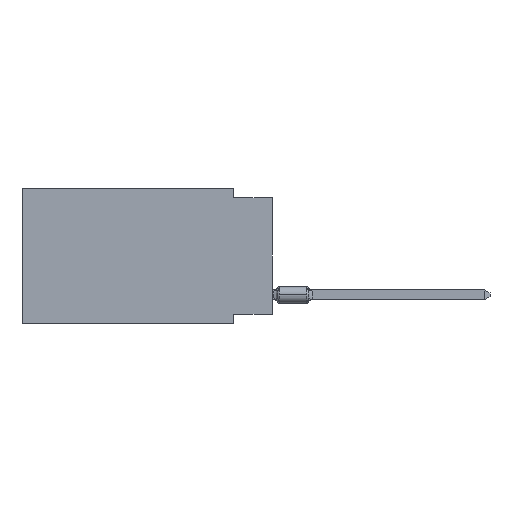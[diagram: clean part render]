
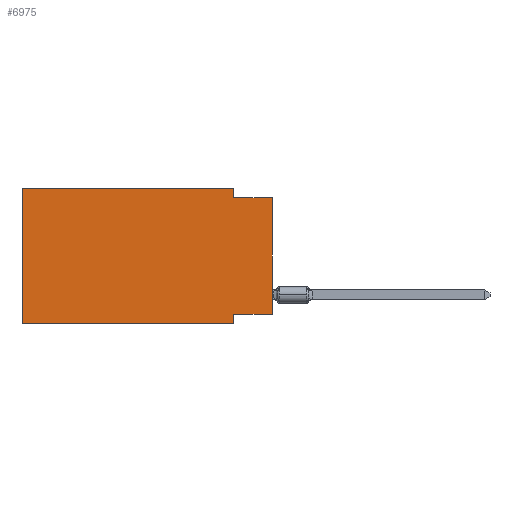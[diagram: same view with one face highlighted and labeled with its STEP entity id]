
A CAD part, left-side view. The second image highlights one B-rep face of the part: STEP entity #6975.
In plain terms, the highlighted planar face has unit normal (-1, 0, 0).
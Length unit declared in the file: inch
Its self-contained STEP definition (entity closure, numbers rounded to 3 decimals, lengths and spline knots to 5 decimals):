
#52 = DIRECTION ( 'NONE',  ( 0., 0., -1. ) ) ;
#82 = CARTESIAN_POINT ( 'NONE',  ( 0., 0.645, -0.35 ) ) ;
#137 = CARTESIAN_POINT ( 'NONE',  ( 0., 0., -0.025 ) ) ;
#347 = VECTOR ( 'NONE', #8689, 39.37008 ) ;
#654 = ORIENTED_EDGE ( 'NONE', *, *, #1019, .T. ) ;
#714 = EDGE_CURVE ( 'NONE', #12337, #725, #11380, .T. ) ;
#725 = VERTEX_POINT ( 'NONE', #10423 ) ;
#746 = VECTOR ( 'NONE', #10069, 39.37008 ) ;
#795 = VECTOR ( 'NONE', #7187, 39.37008 ) ;
#1019 = EDGE_CURVE ( 'NONE', #2766, #12699, #1999, .T. ) ;
#1235 = ORIENTED_EDGE ( 'NONE', *, *, #10185, .F. ) ;
#1402 = EDGE_LOOP ( 'NONE', ( #654, #4165, #5608, #5534, #11131, #13465, #12057, #1235 ) ) ;
#1779 = VERTEX_POINT ( 'NONE', #12945 ) ;
#1970 = EDGE_CURVE ( 'NONE', #10021, #12699, #12278, .T. ) ;
#1999 = LINE ( 'NONE', #2071, #795 ) ;
#2071 = CARTESIAN_POINT ( 'NONE',  ( 0., 0., 0. ) ) ;
#2283 = CARTESIAN_POINT ( 'NONE',  ( 0., 0.645, 0. ) ) ;
#2307 = VECTOR ( 'NONE', #9966, 39.37008 ) ;
#2342 = LINE ( 'NONE', #7653, #347 ) ;
#2606 = CARTESIAN_POINT ( 'NONE',  ( 0., 0.1, 0. ) ) ;
#2766 = VERTEX_POINT ( 'NONE', #10666 ) ;
#3580 = DIRECTION ( 'NONE',  ( 0., -1., 0. ) ) ;
#4165 = ORIENTED_EDGE ( 'NONE', *, *, #1970, .F. ) ;
#4699 = DIRECTION ( 'NONE',  ( 0., 1., 0. ) ) ;
#5534 = ORIENTED_EDGE ( 'NONE', *, *, #10405, .F. ) ;
#5608 = ORIENTED_EDGE ( 'NONE', *, *, #10258, .F. ) ;
#5720 = EDGE_CURVE ( 'NONE', #12337, #11978, #7946, .T. ) ;
#5856 = CARTESIAN_POINT ( 'NONE',  ( 0., 0.1, 0. ) ) ;
#5901 = CARTESIAN_POINT ( 'NONE',  ( 0., 0.645, -0.35 ) ) ;
#5912 = VERTEX_POINT ( 'NONE', #2606 ) ;
#5913 = LINE ( 'NONE', #7006, #7324 ) ;
#5996 = VECTOR ( 'NONE', #10351, 39.37008 ) ;
#6123 = CARTESIAN_POINT ( 'NONE',  ( 0., 0., -0.025 ) ) ;
#6245 = DIRECTION ( 'NONE',  ( 1., 0., 0. ) ) ;
#6637 = CARTESIAN_POINT ( 'NONE',  ( 0., 0.645, 0. ) ) ;
#6774 = LINE ( 'NONE', #6637, #11492 ) ;
#6975 = ADVANCED_FACE ( 'NONE', ( #7466 ), #11645, .F. ) ;
#7006 = CARTESIAN_POINT ( 'NONE',  ( 0., 0., -0.325 ) ) ;
#7187 = DIRECTION ( 'NONE',  ( 0., 0., 1. ) ) ;
#7324 = VECTOR ( 'NONE', #4699, 39.37008 ) ;
#7466 = FACE_OUTER_BOUND ( 'NONE', #1402, .T. ) ;
#7653 = CARTESIAN_POINT ( 'NONE',  ( 0., 0.1, -0.35 ) ) ;
#7946 = LINE ( 'NONE', #5901, #746 ) ;
#8143 = VECTOR ( 'NONE', #10294, 39.37008 ) ;
#8689 = DIRECTION ( 'NONE',  ( 0., 0., -1. ) ) ;
#8693 = EDGE_CURVE ( 'NONE', #1779, #11978, #2342, .T. ) ;
#9228 = AXIS2_PLACEMENT_3D ( 'NONE', #2283, #6245, #52 ) ;
#9534 = CARTESIAN_POINT ( 'NONE',  ( 0., 0.645, 0. ) ) ;
#9618 = CARTESIAN_POINT ( 'NONE',  ( 0., 0.1, -0.025 ) ) ;
#9966 = DIRECTION ( 'NONE',  ( 0., 0., -1. ) ) ;
#10021 = VERTEX_POINT ( 'NONE', #9618 ) ;
#10069 = DIRECTION ( 'NONE',  ( 0., -1., 0. ) ) ;
#10185 = EDGE_CURVE ( 'NONE', #2766, #1779, #5913, .T. ) ;
#10258 = EDGE_CURVE ( 'NONE', #5912, #10021, #13292, .T. ) ;
#10294 = DIRECTION ( 'NONE',  ( 0., -1., 0. ) ) ;
#10351 = DIRECTION ( 'NONE',  ( 0., 0., 1. ) ) ;
#10405 = EDGE_CURVE ( 'NONE', #725, #5912, #6774, .T. ) ;
#10423 = CARTESIAN_POINT ( 'NONE',  ( 0., 0.645, 0. ) ) ;
#10666 = CARTESIAN_POINT ( 'NONE',  ( 0., 0., -0.325 ) ) ;
#11131 = ORIENTED_EDGE ( 'NONE', *, *, #714, .F. ) ;
#11306 = CARTESIAN_POINT ( 'NONE',  ( 0., 0.1, -0.35 ) ) ;
#11380 = LINE ( 'NONE', #9534, #5996 ) ;
#11492 = VECTOR ( 'NONE', #3580, 39.37008 ) ;
#11645 = PLANE ( 'NONE',  #9228 ) ;
#11978 = VERTEX_POINT ( 'NONE', #11306 ) ;
#12057 = ORIENTED_EDGE ( 'NONE', *, *, #8693, .F. ) ;
#12278 = LINE ( 'NONE', #6123, #8143 ) ;
#12337 = VERTEX_POINT ( 'NONE', #82 ) ;
#12699 = VERTEX_POINT ( 'NONE', #137 ) ;
#12945 = CARTESIAN_POINT ( 'NONE',  ( 0., 0.1, -0.325 ) ) ;
#13292 = LINE ( 'NONE', #5856, #2307 ) ;
#13465 = ORIENTED_EDGE ( 'NONE', *, *, #5720, .T. ) ;
